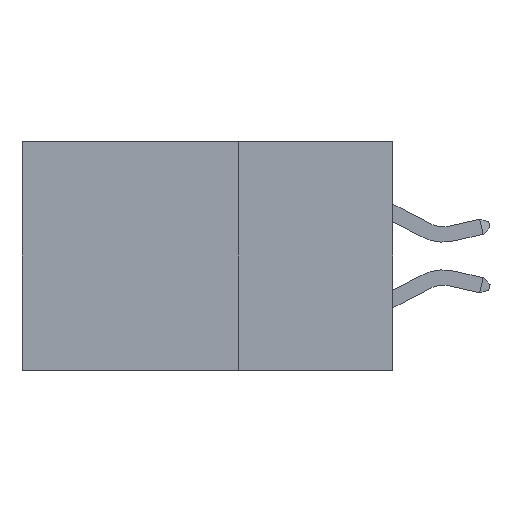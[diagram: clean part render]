
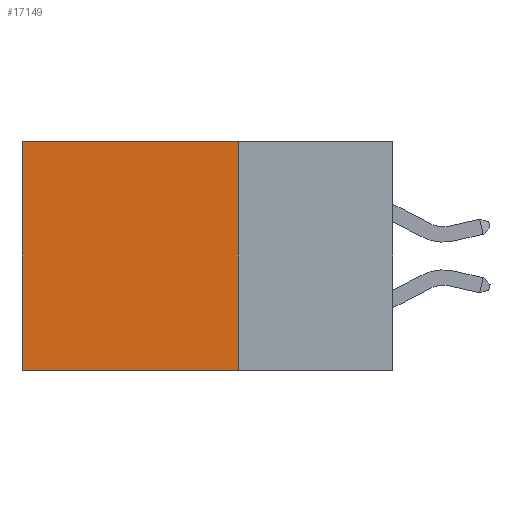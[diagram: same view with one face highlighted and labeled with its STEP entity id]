
A CAD part, left-side view. The second image highlights one B-rep face of the part: STEP entity #17149.
In plain terms, the highlighted planar face has unit normal (-1, 0, 0).
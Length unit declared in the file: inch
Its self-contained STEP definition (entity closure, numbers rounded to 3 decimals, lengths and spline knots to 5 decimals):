
#46 = DIRECTION ( 'NONE',  ( 0., 1., 0. ) ) ;
#408 = CARTESIAN_POINT ( 'NONE',  ( 0.2875, 0.25, -0.37 ) ) ;
#902 = CARTESIAN_POINT ( 'NONE',  ( 0.2875, 0.25, 0. ) ) ;
#910 = CARTESIAN_POINT ( 'NONE',  ( 0.2875, 0.6, 0. ) ) ;
#1099 = EDGE_LOOP ( 'NONE', ( #18051, #14511, #19052, #23607 ) ) ;
#1395 = VERTEX_POINT ( 'NONE', #15475 ) ;
#1894 = VECTOR ( 'NONE', #19950, 39.37008 ) ;
#3840 = VERTEX_POINT ( 'NONE', #902 ) ;
#3909 = CARTESIAN_POINT ( 'NONE',  ( 0.2875, 0.25, 0. ) ) ;
#4000 = LINE ( 'NONE', #3909, #12015 ) ;
#4069 = CARTESIAN_POINT ( 'NONE',  ( 0.2875, 0.25, 0. ) ) ;
#5645 = FACE_OUTER_BOUND ( 'NONE', #1099, .T. ) ;
#6536 = DIRECTION ( 'NONE',  ( 0., 0., -1. ) ) ;
#6767 = EDGE_CURVE ( 'NONE', #3840, #23883, #4000, .T. ) ;
#8189 = VECTOR ( 'NONE', #46, 39.37008 ) ;
#10936 = LINE ( 'NONE', #408, #8189 ) ;
#12015 = VECTOR ( 'NONE', #28139, 39.37008 ) ;
#12023 = DIRECTION ( 'NONE',  ( 0., 0., -1. ) ) ;
#13241 = LINE ( 'NONE', #14348, #28465 ) ;
#14348 = CARTESIAN_POINT ( 'NONE',  ( 0.2875, 0.25, 0. ) ) ;
#14511 = ORIENTED_EDGE ( 'NONE', *, *, #15604, .F. ) ;
#15201 = AXIS2_PLACEMENT_3D ( 'NONE', #4069, #19748, #6536 ) ;
#15425 = PLANE ( 'NONE',  #15201 ) ;
#15475 = CARTESIAN_POINT ( 'NONE',  ( 0.2875, 0.25, -0.37 ) ) ;
#15604 = EDGE_CURVE ( 'NONE', #1395, #19601, #10936, .T. ) ;
#16069 = EDGE_CURVE ( 'NONE', #23883, #19601, #28573, .T. ) ;
#17149 = ADVANCED_FACE ( 'NONE', ( #5645 ), #15425, .F. ) ;
#18051 = ORIENTED_EDGE ( 'NONE', *, *, #16069, .T. ) ;
#19052 = ORIENTED_EDGE ( 'NONE', *, *, #25222, .F. ) ;
#19601 = VERTEX_POINT ( 'NONE', #23328 ) ;
#19748 = DIRECTION ( 'NONE',  ( 1., 0., 0. ) ) ;
#19950 = DIRECTION ( 'NONE',  ( 0., 0., -1. ) ) ;
#23328 = CARTESIAN_POINT ( 'NONE',  ( 0.2875, 0.6, -0.37 ) ) ;
#23607 = ORIENTED_EDGE ( 'NONE', *, *, #6767, .T. ) ;
#23883 = VERTEX_POINT ( 'NONE', #24707 ) ;
#24707 = CARTESIAN_POINT ( 'NONE',  ( 0.2875, 0.6, 0. ) ) ;
#25222 = EDGE_CURVE ( 'NONE', #3840, #1395, #13241, .T. ) ;
#28139 = DIRECTION ( 'NONE',  ( 0., 1., 0. ) ) ;
#28465 = VECTOR ( 'NONE', #12023, 39.37008 ) ;
#28573 = LINE ( 'NONE', #910, #1894 ) ;
